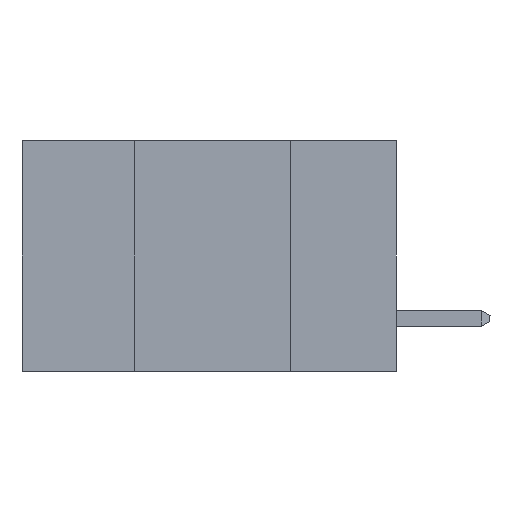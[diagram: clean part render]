
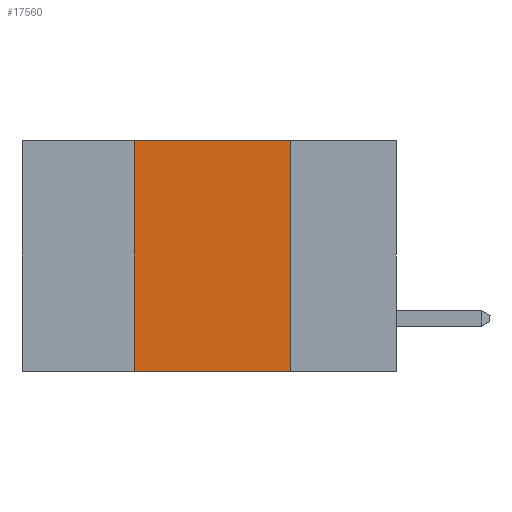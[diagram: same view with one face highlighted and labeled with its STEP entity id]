
A CAD part, left-side view. The second image highlights one B-rep face of the part: STEP entity #17560.
In plain terms, the highlighted planar face has unit normal (-1, 0, 0).
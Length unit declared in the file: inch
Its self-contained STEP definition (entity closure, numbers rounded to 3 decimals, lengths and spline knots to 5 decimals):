
#7 = VECTOR ( 'NONE', #18729, 39.37008 ) ;
#2200 = VECTOR ( 'NONE', #14116, 39.37008 ) ;
#2348 = EDGE_CURVE ( 'NONE', #25026, #25326, #4461, .T. ) ;
#4023 = CARTESIAN_POINT ( 'NONE',  ( 0., 0.6, 0. ) ) ;
#4461 = LINE ( 'NONE', #22939, #7 ) ;
#5139 = AXIS2_PLACEMENT_3D ( 'NONE', #4023, #9599, #7858 ) ;
#5290 = CARTESIAN_POINT ( 'NONE',  ( 0., 0.17, -0.37 ) ) ;
#6728 = VERTEX_POINT ( 'NONE', #22940 ) ;
#7705 = VERTEX_POINT ( 'NONE', #25359 ) ;
#7798 = LINE ( 'NONE', #18343, #15179 ) ;
#7858 = DIRECTION ( 'NONE',  ( 0., 0., -1. ) ) ;
#7983 = PLANE ( 'NONE',  #5139 ) ;
#8872 = ORIENTED_EDGE ( 'NONE', *, *, #14657, .F. ) ;
#9599 = DIRECTION ( 'NONE',  ( 1., 0., 0. ) ) ;
#12171 = DIRECTION ( 'NONE',  ( 0., -1., 0. ) ) ;
#13145 = VECTOR ( 'NONE', #12171, 39.37008 ) ;
#13528 = EDGE_LOOP ( 'NONE', ( #22806, #18953, #8872, #21589 ) ) ;
#14116 = DIRECTION ( 'NONE',  ( 0., 0., -1. ) ) ;
#14208 = FACE_OUTER_BOUND ( 'NONE', #13528, .T. ) ;
#14242 = LINE ( 'NONE', #22259, #2200 ) ;
#14414 = CARTESIAN_POINT ( 'NONE',  ( 0., 0.6, 0. ) ) ;
#14657 = EDGE_CURVE ( 'NONE', #25026, #7705, #7798, .T. ) ;
#15179 = VECTOR ( 'NONE', #16237, 39.37008 ) ;
#16107 = EDGE_CURVE ( 'NONE', #7705, #6728, #20208, .T. ) ;
#16237 = DIRECTION ( 'NONE',  ( 0., 0., 1. ) ) ;
#17560 = ADVANCED_FACE ( 'NONE', ( #14208 ), #7983, .F. ) ;
#18343 = CARTESIAN_POINT ( 'NONE',  ( 0., 0.42, -0.37 ) ) ;
#18477 = EDGE_CURVE ( 'NONE', #6728, #25326, #14242, .T. ) ;
#18729 = DIRECTION ( 'NONE',  ( 0., -1., 0. ) ) ;
#18953 = ORIENTED_EDGE ( 'NONE', *, *, #16107, .F. ) ;
#19828 = CARTESIAN_POINT ( 'NONE',  ( 0., 0.42, -0.37 ) ) ;
#20208 = LINE ( 'NONE', #14414, #13145 ) ;
#21589 = ORIENTED_EDGE ( 'NONE', *, *, #2348, .T. ) ;
#22259 = CARTESIAN_POINT ( 'NONE',  ( 0., 0.17, -0.37 ) ) ;
#22806 = ORIENTED_EDGE ( 'NONE', *, *, #18477, .F. ) ;
#22939 = CARTESIAN_POINT ( 'NONE',  ( 0., 0.6, -0.37 ) ) ;
#22940 = CARTESIAN_POINT ( 'NONE',  ( 0., 0.17, 0. ) ) ;
#25026 = VERTEX_POINT ( 'NONE', #19828 ) ;
#25326 = VERTEX_POINT ( 'NONE', #5290 ) ;
#25359 = CARTESIAN_POINT ( 'NONE',  ( 0., 0.42, 0. ) ) ;
